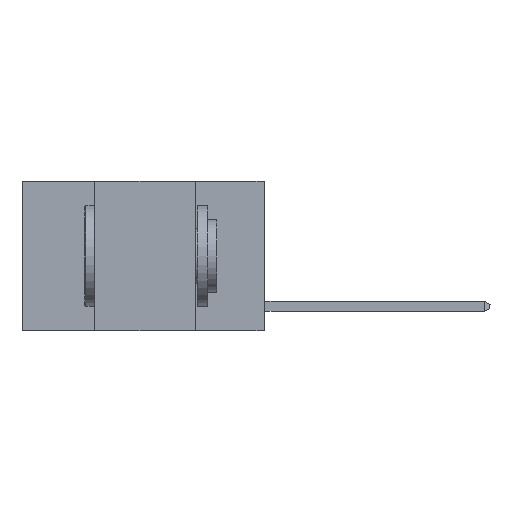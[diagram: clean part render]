
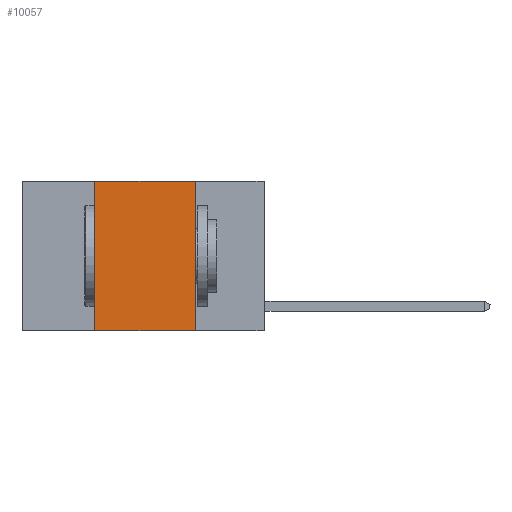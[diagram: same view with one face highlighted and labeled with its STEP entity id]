
A CAD part, left-side view. The second image highlights one B-rep face of the part: STEP entity #10057.
In plain terms, the highlighted planar face has unit normal (-1, 0, 0).
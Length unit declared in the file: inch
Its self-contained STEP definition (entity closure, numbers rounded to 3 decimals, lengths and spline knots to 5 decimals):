
#208 = EDGE_LOOP ( 'NONE', ( #19096, #16052, #8102, #6282 ) ) ;
#1233 = DIRECTION ( 'NONE',  ( 1., 0., 0. ) ) ;
#1947 = DIRECTION ( 'NONE',  ( 0., 0., 1. ) ) ;
#2334 = PLANE ( 'NONE',  #19476 ) ;
#2735 = FACE_OUTER_BOUND ( 'NONE', #208, .T. ) ;
#4651 = LINE ( 'NONE', #9511, #18405 ) ;
#4721 = VECTOR ( 'NONE', #11141, 39.37008 ) ;
#5146 = DIRECTION ( 'NONE',  ( 0., -1., 0. ) ) ;
#5169 = CARTESIAN_POINT ( 'NONE',  ( 0., 0.6, -0.37 ) ) ;
#5337 = CARTESIAN_POINT ( 'NONE',  ( 0., 0.6, 0. ) ) ;
#5745 = VECTOR ( 'NONE', #1947, 39.37008 ) ;
#6103 = LINE ( 'NONE', #12373, #5745 ) ;
#6282 = ORIENTED_EDGE ( 'NONE', *, *, #12983, .T. ) ;
#6398 = CARTESIAN_POINT ( 'NONE',  ( 0., 0.42, -0.37 ) ) ;
#7187 = EDGE_CURVE ( 'NONE', #12216, #8021, #4651, .T. ) ;
#8021 = VERTEX_POINT ( 'NONE', #12291 ) ;
#8102 = ORIENTED_EDGE ( 'NONE', *, *, #16584, .F. ) ;
#8823 = DIRECTION ( 'NONE',  ( 0., 0., -1. ) ) ;
#9511 = CARTESIAN_POINT ( 'NONE',  ( 0., 0.17, 0. ) ) ;
#10057 = ADVANCED_FACE ( 'NONE', ( #2735 ), #2334, .F. ) ;
#11141 = DIRECTION ( 'NONE',  ( 0., -1., 0. ) ) ;
#11348 = VECTOR ( 'NONE', #5146, 39.37008 ) ;
#12173 = VERTEX_POINT ( 'NONE', #15677 ) ;
#12216 = VERTEX_POINT ( 'NONE', #18949 ) ;
#12291 = CARTESIAN_POINT ( 'NONE',  ( 0., 0.17, -0.37 ) ) ;
#12373 = CARTESIAN_POINT ( 'NONE',  ( 0., 0.42, 0. ) ) ;
#12983 = EDGE_CURVE ( 'NONE', #13066, #8021, #18779, .T. ) ;
#13066 = VERTEX_POINT ( 'NONE', #6398 ) ;
#13369 = CARTESIAN_POINT ( 'NONE',  ( 0., 0.6, 0. ) ) ;
#14549 = LINE ( 'NONE', #5337, #11348 ) ;
#15677 = CARTESIAN_POINT ( 'NONE',  ( 0., 0.42, 0. ) ) ;
#16052 = ORIENTED_EDGE ( 'NONE', *, *, #19974, .F. ) ;
#16584 = EDGE_CURVE ( 'NONE', #13066, #12173, #6103, .T. ) ;
#17110 = DIRECTION ( 'NONE',  ( 0., 0., -1. ) ) ;
#18405 = VECTOR ( 'NONE', #17110, 39.37008 ) ;
#18779 = LINE ( 'NONE', #5169, #4721 ) ;
#18949 = CARTESIAN_POINT ( 'NONE',  ( 0., 0.17, 0. ) ) ;
#19096 = ORIENTED_EDGE ( 'NONE', *, *, #7187, .F. ) ;
#19476 = AXIS2_PLACEMENT_3D ( 'NONE', #13369, #1233, #8823 ) ;
#19974 = EDGE_CURVE ( 'NONE', #12173, #12216, #14549, .T. ) ;
